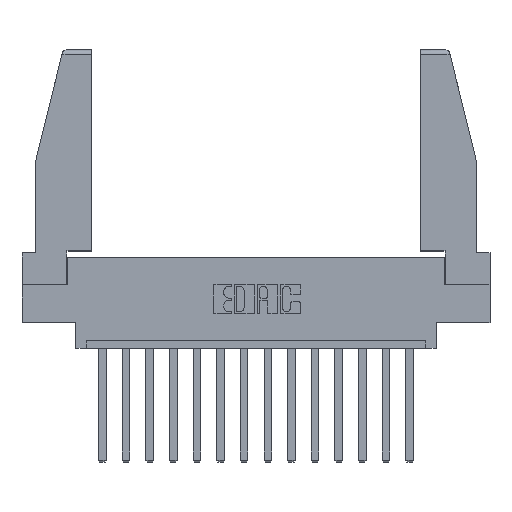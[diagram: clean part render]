
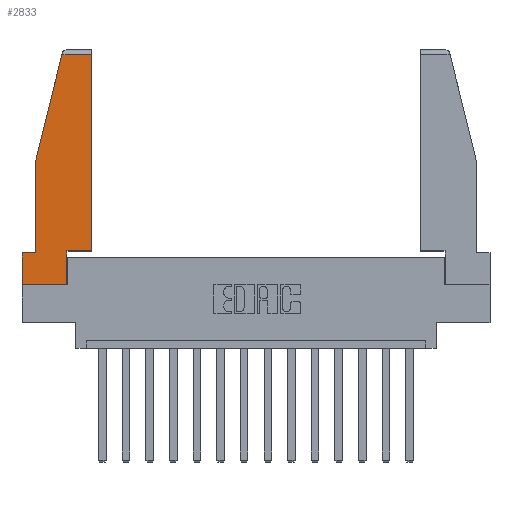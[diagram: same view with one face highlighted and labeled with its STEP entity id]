
A CAD part, top view. The second image highlights one B-rep face of the part: STEP entity #2833.
In plain terms, the highlighted planar face has unit normal (0, 0, 1).
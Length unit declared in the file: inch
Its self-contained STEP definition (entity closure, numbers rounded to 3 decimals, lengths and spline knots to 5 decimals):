
#420 = LINE ( 'NONE', #527, #4623 ) ;
#527 = CARTESIAN_POINT ( 'NONE',  ( 0.086, 0.8, 0. ) ) ;
#551 = DIRECTION ( 'NONE',  ( 0., 1., 0. ) ) ;
#782 = FACE_OUTER_BOUND ( 'NONE', #7811, .T. ) ;
#793 = LINE ( 'NONE', #11795, #2964 ) ;
#1048 = ORIENTED_EDGE ( 'NONE', *, *, #13960, .T. ) ;
#1715 = CARTESIAN_POINT ( 'NONE',  ( 0.297, 0., 0. ) ) ;
#2269 = DIRECTION ( 'NONE',  ( 0., -1., 0. ) ) ;
#2279 = EDGE_CURVE ( 'NONE', #13795, #3406, #3584, .T. ) ;
#2833 = ADVANCED_FACE ( 'NONE', ( #782 ), #6112, .T. ) ;
#2964 = VECTOR ( 'NONE', #9808, 39.37008 ) ;
#3017 = ORIENTED_EDGE ( 'NONE', *, *, #13983, .T. ) ;
#3406 = VERTEX_POINT ( 'NONE', #14932 ) ;
#3584 = LINE ( 'NONE', #16168, #8536 ) ;
#3585 = DIRECTION ( 'NONE',  ( -1., 0., 0. ) ) ;
#3751 = ORIENTED_EDGE ( 'NONE', *, *, #15592, .T. ) ;
#4623 = VECTOR ( 'NONE', #9402, 39.37008 ) ;
#4690 = DIRECTION ( 'NONE',  ( -0.239, -0.971, 0. ) ) ;
#4974 = CARTESIAN_POINT ( 'NONE',  ( 0.461, 0.223, 0. ) ) ;
#5613 = CARTESIAN_POINT ( 'NONE',  ( 0., 0.21, 0. ) ) ;
#5960 = EDGE_CURVE ( 'NONE', #9849, #10792, #15173, .T. ) ;
#6112 = PLANE ( 'NONE',  #15507 ) ;
#6590 = CARTESIAN_POINT ( 'NONE',  ( 0.086, 0.8, 0. ) ) ;
#6761 = CARTESIAN_POINT ( 'NONE',  ( 0.297, 0.223, 0. ) ) ;
#6898 = DIRECTION ( 'NONE',  ( -1., 0., 0. ) ) ;
#7107 = EDGE_CURVE ( 'NONE', #13364, #13795, #15129, .T. ) ;
#7218 = CARTESIAN_POINT ( 'NONE',  ( 0.297, 0., 0. ) ) ;
#7304 = EDGE_CURVE ( 'NONE', #13094, #13364, #420, .T. ) ;
#7609 = ORIENTED_EDGE ( 'NONE', *, *, #9040, .T. ) ;
#7811 = EDGE_LOOP ( 'NONE', ( #16450, #3751, #7609, #15519, #10341, #11021, #3017, #7969, #1048 ) ) ;
#7889 = LINE ( 'NONE', #12203, #12854 ) ;
#7931 = DIRECTION ( 'NONE',  ( 1., 0., 0. ) ) ;
#7969 = ORIENTED_EDGE ( 'NONE', *, *, #5960, .T. ) ;
#8339 = LINE ( 'NONE', #6761, #14687 ) ;
#8536 = VECTOR ( 'NONE', #2269, 39.37008 ) ;
#8703 = CARTESIAN_POINT ( 'NONE',  ( 0.461, 1.52, 0. ) ) ;
#8776 = DIRECTION ( 'NONE',  ( 0., 0., 1. ) ) ;
#9040 = EDGE_CURVE ( 'NONE', #12323, #13094, #7889, .T. ) ;
#9402 = DIRECTION ( 'NONE',  ( 0., -1., 0. ) ) ;
#9706 = LINE ( 'NONE', #11169, #10679 ) ;
#9730 = VERTEX_POINT ( 'NONE', #4974 ) ;
#9808 = DIRECTION ( 'NONE',  ( 1., 0., 0. ) ) ;
#9849 = VERTEX_POINT ( 'NONE', #7218 ) ;
#10207 = CARTESIAN_POINT ( 'NONE',  ( 0., 0.21, 0. ) ) ;
#10341 = ORIENTED_EDGE ( 'NONE', *, *, #7107, .T. ) ;
#10414 = DIRECTION ( 'NONE',  ( 0., 1., 0. ) ) ;
#10475 = CARTESIAN_POINT ( 'NONE',  ( 0.461, 0.223, 0. ) ) ;
#10555 = VECTOR ( 'NONE', #6898, 39.37008 ) ;
#10679 = VECTOR ( 'NONE', #3585, 39.37008 ) ;
#10792 = VERTEX_POINT ( 'NONE', #12346 ) ;
#11021 = ORIENTED_EDGE ( 'NONE', *, *, #2279, .T. ) ;
#11169 = CARTESIAN_POINT ( 'NONE',  ( 0., 1.52, 0. ) ) ;
#11383 = CARTESIAN_POINT ( 'NONE',  ( 0., 0., 0. ) ) ;
#11795 = CARTESIAN_POINT ( 'NONE',  ( 0., 0., 0. ) ) ;
#12203 = CARTESIAN_POINT ( 'NONE',  ( 0.271, 1.55, 0. ) ) ;
#12293 = VERTEX_POINT ( 'NONE', #8703 ) ;
#12323 = VERTEX_POINT ( 'NONE', #15349 ) ;
#12346 = CARTESIAN_POINT ( 'NONE',  ( 0.297, 0.223, 0. ) ) ;
#12854 = VECTOR ( 'NONE', #4690, 39.37008 ) ;
#13094 = VERTEX_POINT ( 'NONE', #6590 ) ;
#13298 = VECTOR ( 'NONE', #10414, 39.37008 ) ;
#13364 = VERTEX_POINT ( 'NONE', #14812 ) ;
#13795 = VERTEX_POINT ( 'NONE', #10207 ) ;
#13960 = EDGE_CURVE ( 'NONE', #10792, #9730, #8339, .T. ) ;
#13983 = EDGE_CURVE ( 'NONE', #3406, #9849, #793, .T. ) ;
#14687 = VECTOR ( 'NONE', #7931, 39.37008 ) ;
#14777 = VECTOR ( 'NONE', #551, 39.37008 ) ;
#14812 = CARTESIAN_POINT ( 'NONE',  ( 0.086, 0.21, 0. ) ) ;
#14861 = EDGE_CURVE ( 'NONE', #9730, #12293, #16069, .T. ) ;
#14932 = CARTESIAN_POINT ( 'NONE',  ( 0., 0., 0. ) ) ;
#15129 = LINE ( 'NONE', #5613, #10555 ) ;
#15173 = LINE ( 'NONE', #1715, #14777 ) ;
#15349 = CARTESIAN_POINT ( 'NONE',  ( 0.2636, 1.52, 0. ) ) ;
#15507 = AXIS2_PLACEMENT_3D ( 'NONE', #11383, #8776, #16211 ) ;
#15519 = ORIENTED_EDGE ( 'NONE', *, *, #7304, .T. ) ;
#15592 = EDGE_CURVE ( 'NONE', #12293, #12323, #9706, .T. ) ;
#16069 = LINE ( 'NONE', #10475, #13298 ) ;
#16168 = CARTESIAN_POINT ( 'NONE',  ( 0., 0.21, 0. ) ) ;
#16211 = DIRECTION ( 'NONE',  ( 1., 0., 0. ) ) ;
#16450 = ORIENTED_EDGE ( 'NONE', *, *, #14861, .T. ) ;
